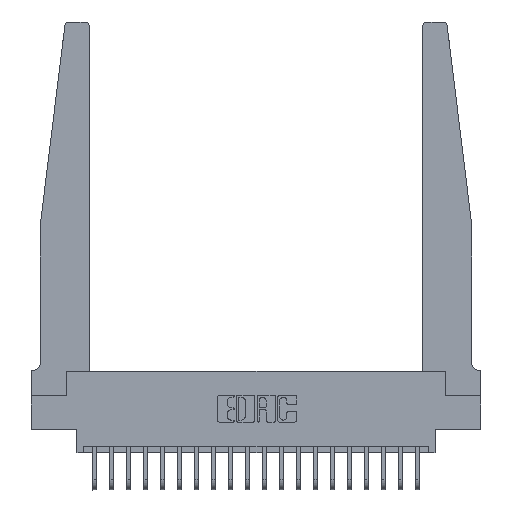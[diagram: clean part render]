
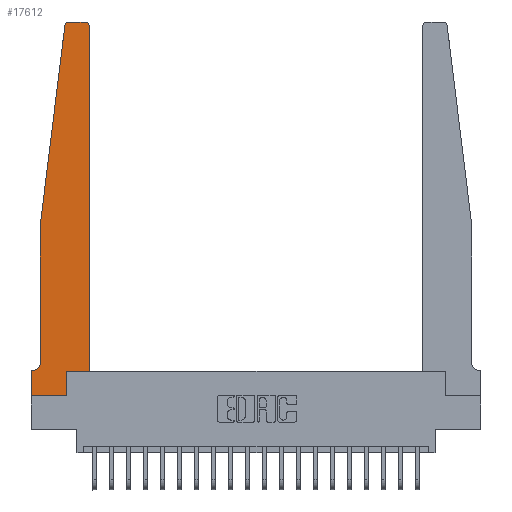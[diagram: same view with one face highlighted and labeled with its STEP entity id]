
A CAD part, top view. The second image highlights one B-rep face of the part: STEP entity #17612.
In plain terms, the highlighted planar face has unit normal (0, 0, 1).
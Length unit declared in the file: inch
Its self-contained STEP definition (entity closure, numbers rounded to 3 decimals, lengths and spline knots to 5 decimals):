
#188 = EDGE_CURVE ( 'NONE', #2283, #18016, #6156, .T. ) ;
#305 = EDGE_CURVE ( 'NONE', #17194, #10071, #13827, .T. ) ;
#609 = VECTOR ( 'NONE', #6000, 39.37008 ) ;
#730 = CARTESIAN_POINT ( 'NONE',  ( 0.425, 0.18, 0.37 ) ) ;
#746 = CARTESIAN_POINT ( 'NONE',  ( 0.2605, 0.18, 0.37 ) ) ;
#1396 = LINE ( 'NONE', #10764, #19472 ) ;
#1427 = CARTESIAN_POINT ( 'NONE',  ( 0.27653, 2.75, 0.37 ) ) ;
#1505 = VECTOR ( 'NONE', #4572, 39.37008 ) ;
#1919 = ORIENTED_EDGE ( 'NONE', *, *, #8591, .T. ) ;
#2175 = CARTESIAN_POINT ( 'NONE',  ( 0.065, 1.25, 0.37 ) ) ;
#2283 = VERTEX_POINT ( 'NONE', #19858 ) ;
#2850 = AXIS2_PLACEMENT_3D ( 'NONE', #16128, #12660, #9394 ) ;
#2912 = DIRECTION ( 'NONE',  ( 1., 0., 0. ) ) ;
#3150 = CARTESIAN_POINT ( 'NONE',  ( 0.25, 2.75, 0.37 ) ) ;
#3663 = VECTOR ( 'NONE', #11705, 39.37008 ) ;
#3749 = VECTOR ( 'NONE', #4811, 39.37008 ) ;
#4572 = DIRECTION ( 'NONE',  ( 0., 1., 0. ) ) ;
#4591 = CARTESIAN_POINT ( 'NONE',  ( 0.065, 0.1875, 0.37 ) ) ;
#4596 = CARTESIAN_POINT ( 'NONE',  ( 0., 0., 0.37 ) ) ;
#4811 = DIRECTION ( 'NONE',  ( -1., 0., 0. ) ) ;
#4934 = DIRECTION ( 'NONE',  ( -1., 0., 0. ) ) ;
#4976 = DIRECTION ( 'NONE',  ( 0., 0., 1. ) ) ;
#5245 = FACE_OUTER_BOUND ( 'NONE', #21186, .T. ) ;
#5257 = EDGE_CURVE ( 'NONE', #20854, #17194, #17744, .T. ) ;
#5542 = LINE ( 'NONE', #7974, #609 ) ;
#5863 = CARTESIAN_POINT ( 'NONE',  ( 0.425, 2.72, 0.37 ) ) ;
#5907 = VERTEX_POINT ( 'NONE', #2175 ) ;
#6000 = DIRECTION ( 'NONE',  ( -0.122, -0.992, 0. ) ) ;
#6156 = LINE ( 'NONE', #746, #1505 ) ;
#6168 = ORIENTED_EDGE ( 'NONE', *, *, #188, .T. ) ;
#6293 = VERTEX_POINT ( 'NONE', #22183 ) ;
#6567 = ORIENTED_EDGE ( 'NONE', *, *, #13344, .T. ) ;
#6952 = DIRECTION ( 'NONE',  ( 0., 0., 1. ) ) ;
#7021 = DIRECTION ( 'NONE',  ( 1., 0., 0. ) ) ;
#7109 = EDGE_CURVE ( 'NONE', #8084, #19044, #16298, .T. ) ;
#7519 = CARTESIAN_POINT ( 'NONE',  ( 0.2605, 0.18, 0.37 ) ) ;
#7742 = EDGE_CURVE ( 'NONE', #18016, #8084, #17622, .T. ) ;
#7839 = CARTESIAN_POINT ( 'NONE',  ( 0., 0.1875, 0.37 ) ) ;
#7974 = CARTESIAN_POINT ( 'NONE',  ( 0.065, 1.25, 0.37 ) ) ;
#8084 = VERTEX_POINT ( 'NONE', #19545 ) ;
#8290 = CARTESIAN_POINT ( 'NONE',  ( 0.425, 0.18, 0.37 ) ) ;
#8591 = EDGE_CURVE ( 'NONE', #17936, #20854, #18840, .T. ) ;
#9394 = DIRECTION ( 'NONE',  ( -1., 0., 0. ) ) ;
#10071 = VERTEX_POINT ( 'NONE', #14761 ) ;
#10521 = CARTESIAN_POINT ( 'NONE',  ( 0.395, 2.72, 0.37 ) ) ;
#10609 = DIRECTION ( 'NONE',  ( 0., -1., 0. ) ) ;
#10764 = CARTESIAN_POINT ( 'NONE',  ( 0.065, 1.25, 0.37 ) ) ;
#11153 = ORIENTED_EDGE ( 'NONE', *, *, #22103, .T. ) ;
#11285 = CARTESIAN_POINT ( 'NONE',  ( 0.24675, 2.72367, 0.37 ) ) ;
#11539 = DIRECTION ( 'NONE',  ( 1., 0., 0. ) ) ;
#11705 = DIRECTION ( 'NONE',  ( 0., -1., 0. ) ) ;
#12283 = AXIS2_PLACEMENT_3D ( 'NONE', #15240, #4976, #18926 ) ;
#12331 = EDGE_CURVE ( 'NONE', #13447, #5907, #5542, .T. ) ;
#12528 = ORIENTED_EDGE ( 'NONE', *, *, #21435, .T. ) ;
#12660 = DIRECTION ( 'NONE',  ( 0., 0., -1. ) ) ;
#13146 = ORIENTED_EDGE ( 'NONE', *, *, #7742, .T. ) ;
#13344 = EDGE_CURVE ( 'NONE', #5907, #17936, #1396, .T. ) ;
#13447 = VERTEX_POINT ( 'NONE', #11285 ) ;
#13827 = LINE ( 'NONE', #4596, #3663 ) ;
#14361 = ORIENTED_EDGE ( 'NONE', *, *, #14414, .T. ) ;
#14414 = EDGE_CURVE ( 'NONE', #10071, #2283, #20809, .T. ) ;
#14513 = ORIENTED_EDGE ( 'NONE', *, *, #5257, .T. ) ;
#14599 = VECTOR ( 'NONE', #2912, 39.37008 ) ;
#14761 = CARTESIAN_POINT ( 'NONE',  ( 0., 0., 0.37 ) ) ;
#14884 = DIRECTION ( 'NONE',  ( 1., 0., 0. ) ) ;
#15184 = VECTOR ( 'NONE', #16523, 39.37008 ) ;
#15240 = CARTESIAN_POINT ( 'NONE',  ( 0.27653, 2.72, 0.37 ) ) ;
#15313 = ORIENTED_EDGE ( 'NONE', *, *, #19387, .T. ) ;
#15516 = CARTESIAN_POINT ( 'NONE',  ( 0., 0.1875, 0.37 ) ) ;
#15594 = VECTOR ( 'NONE', #4934, 39.37008 ) ;
#16128 = CARTESIAN_POINT ( 'NONE',  ( 0.015, 0.2375, 0.37 ) ) ;
#16146 = ORIENTED_EDGE ( 'NONE', *, *, #305, .T. ) ;
#16298 = LINE ( 'NONE', #730, #15184 ) ;
#16523 = DIRECTION ( 'NONE',  ( 0., 1., 0. ) ) ;
#16834 = CIRCLE ( 'NONE', #22481, 0.03 ) ;
#16980 = LINE ( 'NONE', #3150, #15594 ) ;
#17111 = AXIS2_PLACEMENT_3D ( 'NONE', #7839, #20121, #14884 ) ;
#17143 = CIRCLE ( 'NONE', #12283, 0.03 ) ;
#17194 = VERTEX_POINT ( 'NONE', #15516 ) ;
#17511 = CARTESIAN_POINT ( 'NONE',  ( 0.065, 0.2375, 0.37 ) ) ;
#17612 = ADVANCED_FACE ( 'NONE', ( #5245 ), #18364, .T. ) ;
#17622 = LINE ( 'NONE', #8290, #14599 ) ;
#17744 = LINE ( 'NONE', #4591, #3749 ) ;
#17936 = VERTEX_POINT ( 'NONE', #17511 ) ;
#18016 = VERTEX_POINT ( 'NONE', #7519 ) ;
#18364 = PLANE ( 'NONE',  #17111 ) ;
#18691 = ORIENTED_EDGE ( 'NONE', *, *, #7109, .T. ) ;
#18840 = CIRCLE ( 'NONE', #2850, 0.05 ) ;
#18926 = DIRECTION ( 'NONE',  ( 1., 0., 0. ) ) ;
#19044 = VERTEX_POINT ( 'NONE', #5863 ) ;
#19387 = EDGE_CURVE ( 'NONE', #6293, #19487, #16980, .T. ) ;
#19428 = VECTOR ( 'NONE', #11539, 39.37008 ) ;
#19468 = ORIENTED_EDGE ( 'NONE', *, *, #12331, .T. ) ;
#19472 = VECTOR ( 'NONE', #10609, 39.37008 ) ;
#19487 = VERTEX_POINT ( 'NONE', #1427 ) ;
#19545 = CARTESIAN_POINT ( 'NONE',  ( 0.425, 0.18, 0.37 ) ) ;
#19858 = CARTESIAN_POINT ( 'NONE',  ( 0.2605, 0., 0.37 ) ) ;
#20121 = DIRECTION ( 'NONE',  ( 0., 0., 1. ) ) ;
#20525 = CARTESIAN_POINT ( 'NONE',  ( 0., 0., 0.37 ) ) ;
#20809 = LINE ( 'NONE', #20525, #19428 ) ;
#20854 = VERTEX_POINT ( 'NONE', #21026 ) ;
#21026 = CARTESIAN_POINT ( 'NONE',  ( 0.015, 0.1875, 0.37 ) ) ;
#21186 = EDGE_LOOP ( 'NONE', ( #15313, #12528, #19468, #6567, #1919, #14513, #16146, #14361, #6168, #13146, #18691, #11153 ) ) ;
#21435 = EDGE_CURVE ( 'NONE', #19487, #13447, #17143, .T. ) ;
#22103 = EDGE_CURVE ( 'NONE', #19044, #6293, #16834, .T. ) ;
#22183 = CARTESIAN_POINT ( 'NONE',  ( 0.395, 2.75, 0.37 ) ) ;
#22481 = AXIS2_PLACEMENT_3D ( 'NONE', #10521, #6952, #7021 ) ;
